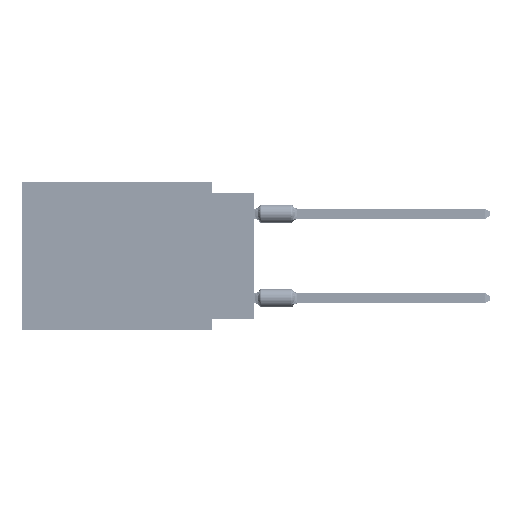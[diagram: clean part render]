
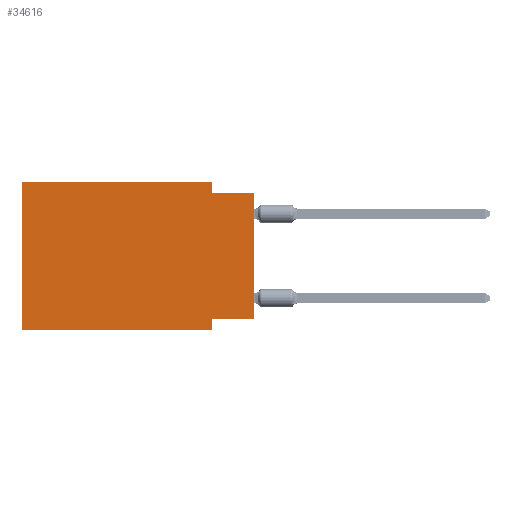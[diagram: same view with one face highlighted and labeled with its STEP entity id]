
A CAD part, left-side view. The second image highlights one B-rep face of the part: STEP entity #34616.
In plain terms, the highlighted planar face has unit normal (-1, 0, 0).
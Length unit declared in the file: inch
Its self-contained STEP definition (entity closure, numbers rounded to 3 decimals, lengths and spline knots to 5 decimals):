
#38 = EDGE_CURVE ( 'NONE', #49933, #57297, #6294, .T. ) ;
#289 = CARTESIAN_POINT ( 'NONE',  ( 0., 0.1, -0.35 ) ) ;
#453 = CARTESIAN_POINT ( 'NONE',  ( 0., 0.55, 0. ) ) ;
#842 = EDGE_CURVE ( 'NONE', #68118, #4644, #14550, .T. ) ;
#1409 = EDGE_CURVE ( 'NONE', #34531, #65672, #49313, .T. ) ;
#1589 = CARTESIAN_POINT ( 'NONE',  ( 0., 0., -0.025 ) ) ;
#2563 = VECTOR ( 'NONE', #33572, 39.37008 ) ;
#3800 = CARTESIAN_POINT ( 'NONE',  ( 0., 0.55, 0. ) ) ;
#4057 = VERTEX_POINT ( 'NONE', #44148 ) ;
#4644 = VERTEX_POINT ( 'NONE', #18543 ) ;
#5922 = DIRECTION ( 'NONE',  ( 0., 0., -1. ) ) ;
#6294 = LINE ( 'NONE', #27980, #2563 ) ;
#8447 = EDGE_CURVE ( 'NONE', #4057, #51498, #37881, .T. ) ;
#9324 = CARTESIAN_POINT ( 'NONE',  ( 0., 0.55, 0. ) ) ;
#9749 = DIRECTION ( 'NONE',  ( 0., 0., -1. ) ) ;
#11180 = CARTESIAN_POINT ( 'NONE',  ( 0., 0.1, 0. ) ) ;
#11510 = DIRECTION ( 'NONE',  ( 0., 0., -1. ) ) ;
#14147 = CARTESIAN_POINT ( 'NONE',  ( 0., 0., 0. ) ) ;
#14481 = EDGE_CURVE ( 'NONE', #51498, #49933, #22026, .T. ) ;
#14550 = LINE ( 'NONE', #32002, #41590 ) ;
#15011 = DIRECTION ( 'NONE',  ( 1., 0., 0. ) ) ;
#16623 = VECTOR ( 'NONE', #5922, 39.37008 ) ;
#18543 = CARTESIAN_POINT ( 'NONE',  ( 0., 0.1, -0.35 ) ) ;
#20259 = PLANE ( 'NONE',  #53088 ) ;
#22026 = LINE ( 'NONE', #11180, #16623 ) ;
#23971 = DIRECTION ( 'NONE',  ( 0., 0., 1. ) ) ;
#27593 = LINE ( 'NONE', #289, #48699 ) ;
#27716 = VECTOR ( 'NONE', #23971, 39.37008 ) ;
#27857 = EDGE_LOOP ( 'NONE', ( #66818, #66853, #65727, #34175, #62672, #67025, #36757, #43377 ) ) ;
#27980 = CARTESIAN_POINT ( 'NONE',  ( 0., 0., -0.025 ) ) ;
#28340 = CARTESIAN_POINT ( 'NONE',  ( 0., 0., -0.325 ) ) ;
#32002 = CARTESIAN_POINT ( 'NONE',  ( 0., 0.55, -0.35 ) ) ;
#33572 = DIRECTION ( 'NONE',  ( 0., -1., 0. ) ) ;
#33586 = DIRECTION ( 'NONE',  ( 0., 1., 0. ) ) ;
#34175 = ORIENTED_EDGE ( 'NONE', *, *, #8447, .F. ) ;
#34531 = VERTEX_POINT ( 'NONE', #56603 ) ;
#34616 = ADVANCED_FACE ( 'NONE', ( #51695 ), #20259, .F. ) ;
#36757 = ORIENTED_EDGE ( 'NONE', *, *, #37159, .F. ) ;
#37159 = EDGE_CURVE ( 'NONE', #65672, #4644, #27593, .T. ) ;
#37251 = DIRECTION ( 'NONE',  ( 0., -1., 0. ) ) ;
#37881 = LINE ( 'NONE', #453, #39339 ) ;
#39339 = VECTOR ( 'NONE', #43124, 39.37008 ) ;
#40039 = EDGE_CURVE ( 'NONE', #68118, #4057, #46380, .T. ) ;
#41590 = VECTOR ( 'NONE', #37251, 39.37008 ) ;
#42046 = CARTESIAN_POINT ( 'NONE',  ( 0., 0.1, 0. ) ) ;
#43124 = DIRECTION ( 'NONE',  ( 0., -1., 0. ) ) ;
#43377 = ORIENTED_EDGE ( 'NONE', *, *, #1409, .F. ) ;
#43841 = CARTESIAN_POINT ( 'NONE',  ( 0., 0.1, -0.025 ) ) ;
#43899 = VECTOR ( 'NONE', #33586, 39.37008 ) ;
#44148 = CARTESIAN_POINT ( 'NONE',  ( 0., 0.55, 0. ) ) ;
#46045 = DIRECTION ( 'NONE',  ( 0., 0., 1. ) ) ;
#46380 = LINE ( 'NONE', #9324, #56817 ) ;
#48401 = EDGE_CURVE ( 'NONE', #34531, #57297, #67954, .T. ) ;
#48699 = VECTOR ( 'NONE', #11510, 39.37008 ) ;
#49313 = LINE ( 'NONE', #28340, #43899 ) ;
#49933 = VERTEX_POINT ( 'NONE', #43841 ) ;
#51498 = VERTEX_POINT ( 'NONE', #42046 ) ;
#51695 = FACE_OUTER_BOUND ( 'NONE', #27857, .T. ) ;
#53088 = AXIS2_PLACEMENT_3D ( 'NONE', #3800, #15011, #9749 ) ;
#56603 = CARTESIAN_POINT ( 'NONE',  ( 0., 0., -0.325 ) ) ;
#56817 = VECTOR ( 'NONE', #46045, 39.37008 ) ;
#57297 = VERTEX_POINT ( 'NONE', #1589 ) ;
#62672 = ORIENTED_EDGE ( 'NONE', *, *, #40039, .F. ) ;
#63232 = CARTESIAN_POINT ( 'NONE',  ( 0., 0.1, -0.325 ) ) ;
#65672 = VERTEX_POINT ( 'NONE', #63232 ) ;
#65727 = ORIENTED_EDGE ( 'NONE', *, *, #14481, .F. ) ;
#66818 = ORIENTED_EDGE ( 'NONE', *, *, #48401, .T. ) ;
#66853 = ORIENTED_EDGE ( 'NONE', *, *, #38, .F. ) ;
#67025 = ORIENTED_EDGE ( 'NONE', *, *, #842, .T. ) ;
#67954 = LINE ( 'NONE', #14147, #27716 ) ;
#68118 = VERTEX_POINT ( 'NONE', #68854 ) ;
#68854 = CARTESIAN_POINT ( 'NONE',  ( 0., 0.55, -0.35 ) ) ;
